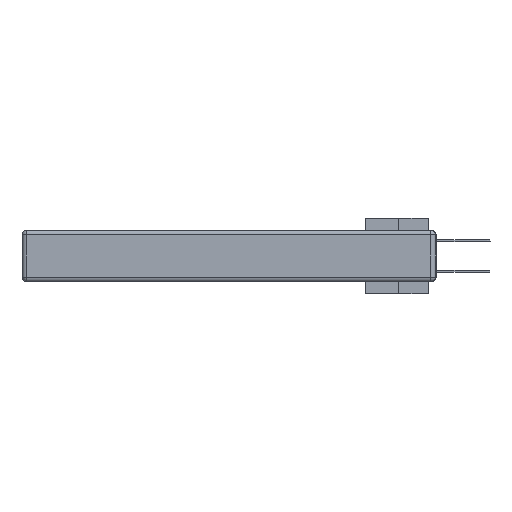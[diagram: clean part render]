
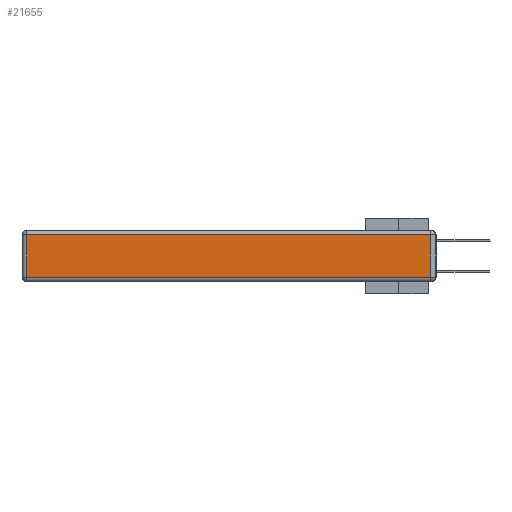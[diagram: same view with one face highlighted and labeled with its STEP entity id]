
A CAD part, left-side view. The second image highlights one B-rep face of the part: STEP entity #21655.
In plain terms, the highlighted planar face has unit normal (-1, 0, 0).
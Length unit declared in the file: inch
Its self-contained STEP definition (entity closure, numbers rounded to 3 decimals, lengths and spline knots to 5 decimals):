
#1657 = LINE ( 'NONE', #19643, #11148 ) ;
#3239 = EDGE_CURVE ( 'NONE', #23713, #11332, #1657, .T. ) ;
#3467 = CARTESIAN_POINT ( 'NONE',  ( 0., 0.03, -0.03 ) ) ;
#3544 = CARTESIAN_POINT ( 'NONE',  ( 0., 0., -0.313 ) ) ;
#4932 = DIRECTION ( 'NONE',  ( -1., 0., 0. ) ) ;
#5671 = ORIENTED_EDGE ( 'NONE', *, *, #3239, .T. ) ;
#7155 = CARTESIAN_POINT ( 'NONE',  ( 0., 0.03, -0.313 ) ) ;
#7282 = CARTESIAN_POINT ( 'NONE',  ( 0., 0., -0.343 ) ) ;
#8993 = CARTESIAN_POINT ( 'NONE',  ( 0., 2.72, -0.03 ) ) ;
#9299 = EDGE_CURVE ( 'NONE', #21150, #24595, #16187, .T. ) ;
#10628 = VECTOR ( 'NONE', #11317, 39.37008 ) ;
#10949 = ORIENTED_EDGE ( 'NONE', *, *, #11736, .T. ) ;
#11148 = VECTOR ( 'NONE', #29713, 39.37008 ) ;
#11317 = DIRECTION ( 'NONE',  ( 0., -1., 0. ) ) ;
#11332 = VERTEX_POINT ( 'NONE', #22678 ) ;
#11736 = EDGE_CURVE ( 'NONE', #24595, #23713, #22639, .T. ) ;
#14154 = LINE ( 'NONE', #3544, #10628 ) ;
#16029 = EDGE_CURVE ( 'NONE', #11332, #21150, #14154, .T. ) ;
#16187 = LINE ( 'NONE', #26106, #26213 ) ;
#16322 = ORIENTED_EDGE ( 'NONE', *, *, #9299, .T. ) ;
#18301 = AXIS2_PLACEMENT_3D ( 'NONE', #7282, #4932, #25265 ) ;
#19643 = CARTESIAN_POINT ( 'NONE',  ( 0., 2.72, -0.343 ) ) ;
#20076 = ORIENTED_EDGE ( 'NONE', *, *, #16029, .T. ) ;
#20440 = DIRECTION ( 'NONE',  ( 0., 1., 0. ) ) ;
#21150 = VERTEX_POINT ( 'NONE', #7155 ) ;
#21655 = ADVANCED_FACE ( 'NONE', ( #32803 ), #30285, .T. ) ;
#22639 = LINE ( 'NONE', #32876, #32060 ) ;
#22678 = CARTESIAN_POINT ( 'NONE',  ( 0., 2.72, -0.313 ) ) ;
#23713 = VERTEX_POINT ( 'NONE', #8993 ) ;
#24595 = VERTEX_POINT ( 'NONE', #3467 ) ;
#25265 = DIRECTION ( 'NONE',  ( 0., 0., 1. ) ) ;
#26106 = CARTESIAN_POINT ( 'NONE',  ( 0., 0.03, -0.343 ) ) ;
#26213 = VECTOR ( 'NONE', #30523, 39.37008 ) ;
#28720 = EDGE_LOOP ( 'NONE', ( #20076, #16322, #10949, #5671 ) ) ;
#29713 = DIRECTION ( 'NONE',  ( 0., 0., -1. ) ) ;
#30285 = PLANE ( 'NONE',  #18301 ) ;
#30523 = DIRECTION ( 'NONE',  ( 0., 0., 1. ) ) ;
#32060 = VECTOR ( 'NONE', #20440, 39.37008 ) ;
#32803 = FACE_OUTER_BOUND ( 'NONE', #28720, .T. ) ;
#32876 = CARTESIAN_POINT ( 'NONE',  ( 0., 2.75, -0.03 ) ) ;
